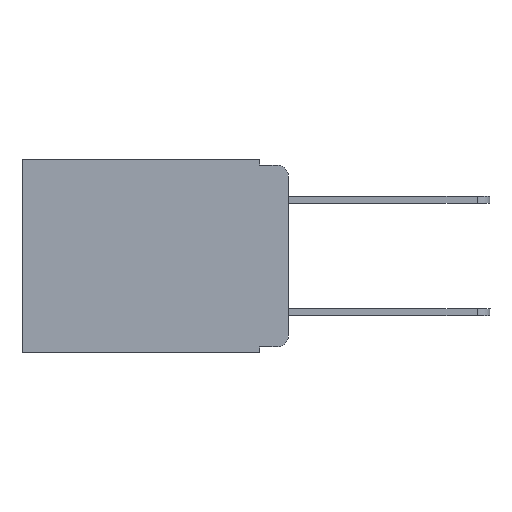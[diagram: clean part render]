
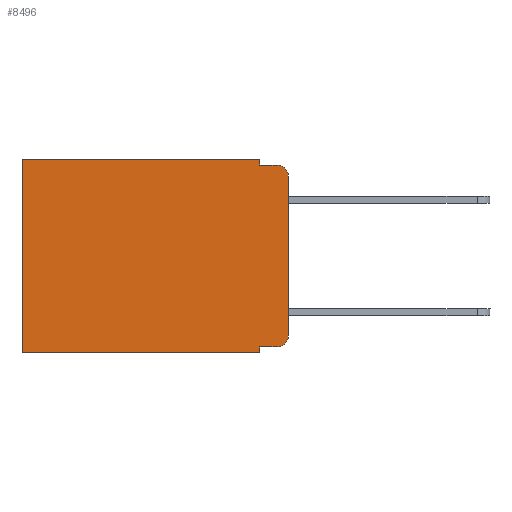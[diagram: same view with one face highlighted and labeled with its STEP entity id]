
A CAD part, left-side view. The second image highlights one B-rep face of the part: STEP entity #8496.
In plain terms, the highlighted planar face has unit normal (-1, 0, 0).
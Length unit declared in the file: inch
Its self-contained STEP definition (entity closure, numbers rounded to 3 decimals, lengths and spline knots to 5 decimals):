
#108 = LINE ( 'NONE', #5912, #6100 ) ;
#170 = CARTESIAN_POINT ( 'NONE',  ( 0.298, 0.473, 0. ) ) ;
#203 = ORIENTED_EDGE ( 'NONE', *, *, #2074, .T. ) ;
#439 = CARTESIAN_POINT ( 'NONE',  ( 0.298, 0., -0.313 ) ) ;
#576 = DIRECTION ( 'NONE',  ( 0., 0., -1. ) ) ;
#747 = VERTEX_POINT ( 'NONE', #1489 ) ;
#841 = DIRECTION ( 'NONE',  ( 0., 0., -1. ) ) ;
#1144 = AXIS2_PLACEMENT_3D ( 'NONE', #8821, #5312, #6618 ) ;
#1221 = LINE ( 'NONE', #3781, #4994 ) ;
#1222 = VERTEX_POINT ( 'NONE', #8383 ) ;
#1232 = ORIENTED_EDGE ( 'NONE', *, *, #4956, .T. ) ;
#1276 = CARTESIAN_POINT ( 'NONE',  ( 0.298, 0.02, -0.01 ) ) ;
#1288 = VECTOR ( 'NONE', #3520, 39.37008 ) ;
#1351 = CARTESIAN_POINT ( 'NONE',  ( 0.298, 0.473, 0. ) ) ;
#1489 = CARTESIAN_POINT ( 'NONE',  ( 0.298, 0.051, -0.333 ) ) ;
#1560 = EDGE_CURVE ( 'NONE', #747, #5124, #2215, .T. ) ;
#1731 = ORIENTED_EDGE ( 'NONE', *, *, #5542, .T. ) ;
#1747 = EDGE_LOOP ( 'NONE', ( #7547, #5252, #3118, #8237, #203, #8612, #8738, #3220, #1232, #1731 ) ) ;
#2074 = EDGE_CURVE ( 'NONE', #9226, #9065, #6551, .T. ) ;
#2215 = LINE ( 'NONE', #5170, #1288 ) ;
#2433 = VERTEX_POINT ( 'NONE', #4364 ) ;
#2492 = PLANE ( 'NONE',  #8211 ) ;
#2979 = CIRCLE ( 'NONE', #1144, 0.02 ) ;
#2985 = CARTESIAN_POINT ( 'NONE',  ( 0.298, 0., 0. ) ) ;
#3118 = ORIENTED_EDGE ( 'NONE', *, *, #3763, .F. ) ;
#3220 = ORIENTED_EDGE ( 'NONE', *, *, #1560, .F. ) ;
#3512 = CIRCLE ( 'NONE', #7056, 0.02 ) ;
#3520 = DIRECTION ( 'NONE',  ( 0., 0., -1. ) ) ;
#3635 = CARTESIAN_POINT ( 'NONE',  ( 0.298, 0.02, -0.313 ) ) ;
#3763 = EDGE_CURVE ( 'NONE', #7879, #5783, #108, .T. ) ;
#3781 = CARTESIAN_POINT ( 'NONE',  ( 0.298, 0.051, -0.333 ) ) ;
#3801 = VECTOR ( 'NONE', #576, 39.37008 ) ;
#4334 = LINE ( 'NONE', #170, #6830 ) ;
#4364 = CARTESIAN_POINT ( 'NONE',  ( 0.298, 0., -0.03 ) ) ;
#4725 = CARTESIAN_POINT ( 'NONE',  ( 0.298, 0., 0. ) ) ;
#4848 = LINE ( 'NONE', #9391, #3801 ) ;
#4956 = EDGE_CURVE ( 'NONE', #747, #1222, #1221, .T. ) ;
#4994 = VECTOR ( 'NONE', #6727, 39.37008 ) ;
#5124 = VERTEX_POINT ( 'NONE', #6922 ) ;
#5170 = CARTESIAN_POINT ( 'NONE',  ( 0.298, 0.051, 0. ) ) ;
#5193 = CARTESIAN_POINT ( 'NONE',  ( 0.298, 0.051, 0. ) ) ;
#5252 = ORIENTED_EDGE ( 'NONE', *, *, #6605, .T. ) ;
#5278 = EDGE_CURVE ( 'NONE', #2433, #7779, #4848, .T. ) ;
#5280 = DIRECTION ( 'NONE',  ( 0., -1., 0. ) ) ;
#5303 = LINE ( 'NONE', #7420, #6672 ) ;
#5312 = DIRECTION ( 'NONE',  ( -1., 0., 0. ) ) ;
#5394 = DIRECTION ( 'NONE',  ( 0., 0., -1. ) ) ;
#5529 = CARTESIAN_POINT ( 'NONE',  ( 0.298, 0.473, -0.343 ) ) ;
#5542 = EDGE_CURVE ( 'NONE', #1222, #7779, #3512, .T. ) ;
#5783 = VERTEX_POINT ( 'NONE', #1276 ) ;
#5912 = CARTESIAN_POINT ( 'NONE',  ( 0.298, 0.051, -0.01 ) ) ;
#6100 = VECTOR ( 'NONE', #5280, 39.37008 ) ;
#6194 = DIRECTION ( 'NONE',  ( 0., 1., 0. ) ) ;
#6551 = LINE ( 'NONE', #2985, #6984 ) ;
#6605 = EDGE_CURVE ( 'NONE', #2433, #5783, #2979, .T. ) ;
#6618 = DIRECTION ( 'NONE',  ( 0., 0., -1. ) ) ;
#6672 = VECTOR ( 'NONE', #841, 39.37008 ) ;
#6727 = DIRECTION ( 'NONE',  ( 0., -1., 0. ) ) ;
#6830 = VECTOR ( 'NONE', #8903, 39.37008 ) ;
#6922 = CARTESIAN_POINT ( 'NONE',  ( 0.298, 0.051, -0.343 ) ) ;
#6984 = VECTOR ( 'NONE', #8854, 39.37008 ) ;
#7045 = EDGE_CURVE ( 'NONE', #9065, #9026, #4334, .T. ) ;
#7056 = AXIS2_PLACEMENT_3D ( 'NONE', #3635, #7534, #8443 ) ;
#7303 = CARTESIAN_POINT ( 'NONE',  ( 0.298, 0.051, -0.01 ) ) ;
#7307 = VECTOR ( 'NONE', #6194, 39.37008 ) ;
#7420 = CARTESIAN_POINT ( 'NONE',  ( 0.298, 0.051, 0. ) ) ;
#7534 = DIRECTION ( 'NONE',  ( -1., 0., 0. ) ) ;
#7547 = ORIENTED_EDGE ( 'NONE', *, *, #5278, .F. ) ;
#7668 = EDGE_CURVE ( 'NONE', #5124, #9026, #8356, .T. ) ;
#7672 = DIRECTION ( 'NONE',  ( 1., 0., 0. ) ) ;
#7779 = VERTEX_POINT ( 'NONE', #439 ) ;
#7879 = VERTEX_POINT ( 'NONE', #7303 ) ;
#8211 = AXIS2_PLACEMENT_3D ( 'NONE', #4725, #7672, #5394 ) ;
#8237 = ORIENTED_EDGE ( 'NONE', *, *, #8375, .F. ) ;
#8356 = LINE ( 'NONE', #9125, #7307 ) ;
#8373 = FACE_OUTER_BOUND ( 'NONE', #1747, .T. ) ;
#8375 = EDGE_CURVE ( 'NONE', #9226, #7879, #5303, .T. ) ;
#8383 = CARTESIAN_POINT ( 'NONE',  ( 0.298, 0.02, -0.333 ) ) ;
#8443 = DIRECTION ( 'NONE',  ( 0., 0., -1. ) ) ;
#8496 = ADVANCED_FACE ( 'NONE', ( #8373 ), #2492, .F. ) ;
#8612 = ORIENTED_EDGE ( 'NONE', *, *, #7045, .T. ) ;
#8738 = ORIENTED_EDGE ( 'NONE', *, *, #7668, .F. ) ;
#8821 = CARTESIAN_POINT ( 'NONE',  ( 0.298, 0.02, -0.03 ) ) ;
#8854 = DIRECTION ( 'NONE',  ( 0., 1., 0. ) ) ;
#8903 = DIRECTION ( 'NONE',  ( 0., 0., -1. ) ) ;
#9026 = VERTEX_POINT ( 'NONE', #5529 ) ;
#9065 = VERTEX_POINT ( 'NONE', #1351 ) ;
#9125 = CARTESIAN_POINT ( 'NONE',  ( 0.298, 0., -0.343 ) ) ;
#9226 = VERTEX_POINT ( 'NONE', #5193 ) ;
#9391 = CARTESIAN_POINT ( 'NONE',  ( 0.298, 0., 0. ) ) ;
